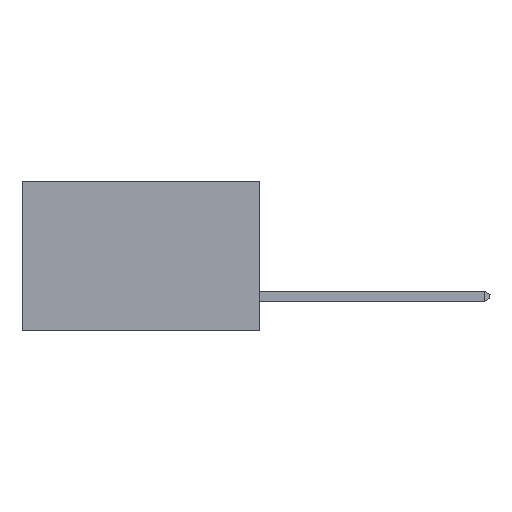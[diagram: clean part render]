
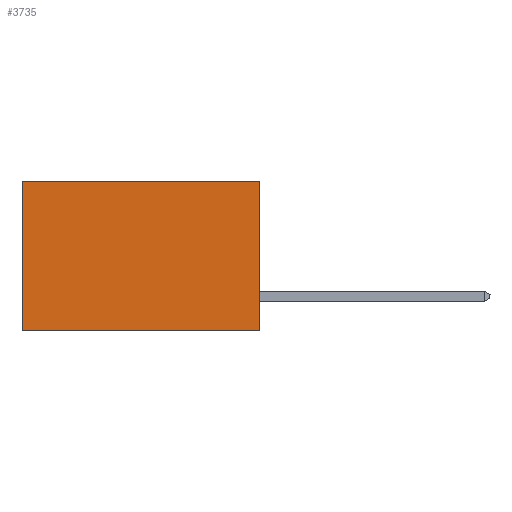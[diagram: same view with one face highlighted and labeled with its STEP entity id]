
A CAD part, left-side view. The second image highlights one B-rep face of the part: STEP entity #3735.
In plain terms, the highlighted planar face has unit normal (-1, 0, 0).
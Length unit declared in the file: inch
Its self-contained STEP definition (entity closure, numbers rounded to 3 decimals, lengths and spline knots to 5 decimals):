
#127 = EDGE_CURVE ( 'NONE', #6070, #1120, #9296, .T. ) ;
#273 = CARTESIAN_POINT ( 'NONE',  ( 0.277, 0., 0. ) ) ;
#331 = CARTESIAN_POINT ( 'NONE',  ( 0.277, 0.59, -0.37 ) ) ;
#341 = DIRECTION ( 'NONE',  ( 0., 1., 0. ) ) ;
#640 = EDGE_CURVE ( 'NONE', #8135, #6070, #8260, .T. ) ;
#1120 = VERTEX_POINT ( 'NONE', #331 ) ;
#1237 = VECTOR ( 'NONE', #9845, 39.37008 ) ;
#1451 = EDGE_CURVE ( 'NONE', #7654, #1120, #8133, .T. ) ;
#1721 = CARTESIAN_POINT ( 'NONE',  ( 0.277, 0., -0.37 ) ) ;
#1769 = CARTESIAN_POINT ( 'NONE',  ( 0.277, 0.59, 0. ) ) ;
#2884 = LINE ( 'NONE', #273, #5113 ) ;
#3088 = ORIENTED_EDGE ( 'NONE', *, *, #1451, .T. ) ;
#3284 = DIRECTION ( 'NONE',  ( 1., 0., 0. ) ) ;
#3735 = ADVANCED_FACE ( 'NONE', ( #6411 ), #10021, .F. ) ;
#4270 = AXIS2_PLACEMENT_3D ( 'NONE', #4911, #3284, #4626 ) ;
#4288 = CARTESIAN_POINT ( 'NONE',  ( 0.277, 0., -0.37 ) ) ;
#4356 = DIRECTION ( 'NONE',  ( 0., 1., 0. ) ) ;
#4626 = DIRECTION ( 'NONE',  ( 0., 0., -1. ) ) ;
#4911 = CARTESIAN_POINT ( 'NONE',  ( 0.277, 0., -0.37 ) ) ;
#5113 = VECTOR ( 'NONE', #341, 39.37008 ) ;
#5927 = CARTESIAN_POINT ( 'NONE',  ( 0.277, 0., 0. ) ) ;
#6070 = VERTEX_POINT ( 'NONE', #8178 ) ;
#6097 = VECTOR ( 'NONE', #8335, 39.37008 ) ;
#6411 = FACE_OUTER_BOUND ( 'NONE', #8869, .T. ) ;
#6875 = CARTESIAN_POINT ( 'NONE',  ( 0.277, 0.59, -0.37 ) ) ;
#6912 = VECTOR ( 'NONE', #4356, 39.37008 ) ;
#7196 = ORIENTED_EDGE ( 'NONE', *, *, #8497, .T. ) ;
#7654 = VERTEX_POINT ( 'NONE', #1769 ) ;
#8133 = LINE ( 'NONE', #6875, #1237 ) ;
#8135 = VERTEX_POINT ( 'NONE', #5927 ) ;
#8160 = ORIENTED_EDGE ( 'NONE', *, *, #640, .F. ) ;
#8178 = CARTESIAN_POINT ( 'NONE',  ( 0.277, 0., -0.37 ) ) ;
#8260 = LINE ( 'NONE', #1721, #6097 ) ;
#8335 = DIRECTION ( 'NONE',  ( 0., 0., -1. ) ) ;
#8497 = EDGE_CURVE ( 'NONE', #8135, #7654, #2884, .T. ) ;
#8869 = EDGE_LOOP ( 'NONE', ( #3088, #9955, #8160, #7196 ) ) ;
#9296 = LINE ( 'NONE', #4288, #6912 ) ;
#9845 = DIRECTION ( 'NONE',  ( 0., 0., -1. ) ) ;
#9955 = ORIENTED_EDGE ( 'NONE', *, *, #127, .F. ) ;
#10021 = PLANE ( 'NONE',  #4270 ) ;
